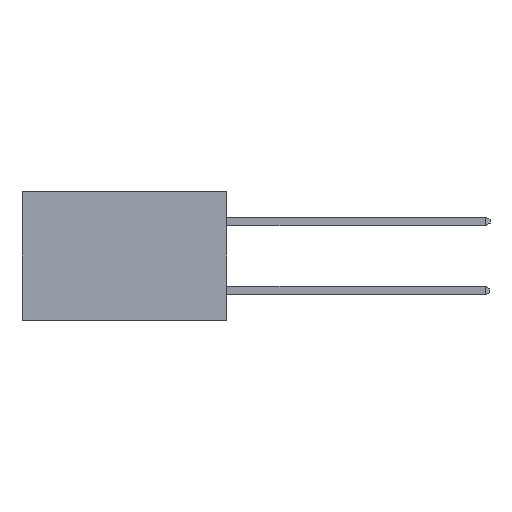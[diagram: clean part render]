
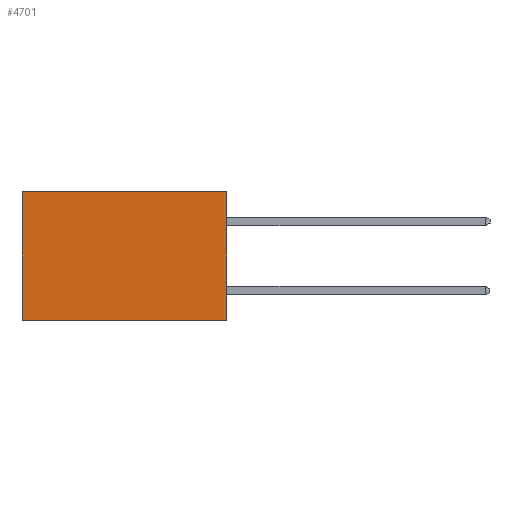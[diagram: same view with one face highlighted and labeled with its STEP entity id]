
A CAD part, left-side view. The second image highlights one B-rep face of the part: STEP entity #4701.
In plain terms, the highlighted planar face has unit normal (-1, 0, 0).
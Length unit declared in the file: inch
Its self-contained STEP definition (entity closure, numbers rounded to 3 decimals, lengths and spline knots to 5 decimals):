
#24 = CARTESIAN_POINT ( 'NONE',  ( 0.277, 0., -0.37 ) ) ;
#373 = CARTESIAN_POINT ( 'NONE',  ( 0.277, 0.59, 0. ) ) ;
#494 = LINE ( 'NONE', #24, #2741 ) ;
#520 = PLANE ( 'NONE',  #6281 ) ;
#527 = CARTESIAN_POINT ( 'NONE',  ( 0.277, 0.59, -0.37 ) ) ;
#631 = DIRECTION ( 'NONE',  ( 0., 0., -1. ) ) ;
#736 = VECTOR ( 'NONE', #6681, 39.37008 ) ;
#1031 = DIRECTION ( 'NONE',  ( 1., 0., 0. ) ) ;
#1507 = CARTESIAN_POINT ( 'NONE',  ( 0.277, 0., -0.37 ) ) ;
#2441 = ORIENTED_EDGE ( 'NONE', *, *, #7506, .T. ) ;
#2741 = VECTOR ( 'NONE', #12286, 39.37008 ) ;
#3644 = LINE ( 'NONE', #8388, #9407 ) ;
#3730 = EDGE_CURVE ( 'NONE', #10441, #4803, #3644, .T. ) ;
#4040 = ORIENTED_EDGE ( 'NONE', *, *, #13483, .F. ) ;
#4305 = ORIENTED_EDGE ( 'NONE', *, *, #3730, .F. ) ;
#4465 = LINE ( 'NONE', #9948, #736 ) ;
#4701 = ADVANCED_FACE ( 'NONE', ( #10390 ), #520, .F. ) ;
#4711 = VERTEX_POINT ( 'NONE', #373 ) ;
#4803 = VERTEX_POINT ( 'NONE', #10119 ) ;
#6050 = EDGE_LOOP ( 'NONE', ( #8734, #4040, #4305, #2441 ) ) ;
#6281 = AXIS2_PLACEMENT_3D ( 'NONE', #1507, #1031, #631 ) ;
#6681 = DIRECTION ( 'NONE',  ( 0., 1., 0. ) ) ;
#6859 = VERTEX_POINT ( 'NONE', #527 ) ;
#7506 = EDGE_CURVE ( 'NONE', #10441, #4711, #4465, .T. ) ;
#8388 = CARTESIAN_POINT ( 'NONE',  ( 0.277, 0., -0.37 ) ) ;
#8734 = ORIENTED_EDGE ( 'NONE', *, *, #10019, .T. ) ;
#9407 = VECTOR ( 'NONE', #12108, 39.37008 ) ;
#9627 = CARTESIAN_POINT ( 'NONE',  ( 0.277, 0., 0. ) ) ;
#9922 = CARTESIAN_POINT ( 'NONE',  ( 0.277, 0.59, -0.37 ) ) ;
#9948 = CARTESIAN_POINT ( 'NONE',  ( 0.277, 0., 0. ) ) ;
#10019 = EDGE_CURVE ( 'NONE', #4711, #6859, #14048, .T. ) ;
#10119 = CARTESIAN_POINT ( 'NONE',  ( 0.277, 0., -0.37 ) ) ;
#10390 = FACE_OUTER_BOUND ( 'NONE', #6050, .T. ) ;
#10441 = VERTEX_POINT ( 'NONE', #9627 ) ;
#11486 = VECTOR ( 'NONE', #13930, 39.37008 ) ;
#12108 = DIRECTION ( 'NONE',  ( 0., 0., -1. ) ) ;
#12286 = DIRECTION ( 'NONE',  ( 0., 1., 0. ) ) ;
#13483 = EDGE_CURVE ( 'NONE', #4803, #6859, #494, .T. ) ;
#13930 = DIRECTION ( 'NONE',  ( 0., 0., -1. ) ) ;
#14048 = LINE ( 'NONE', #9922, #11486 ) ;
